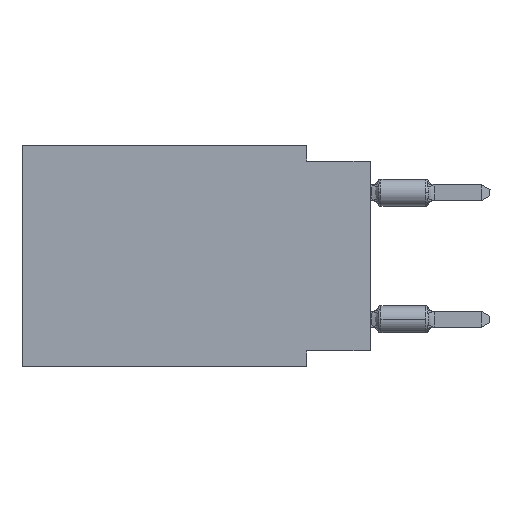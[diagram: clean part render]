
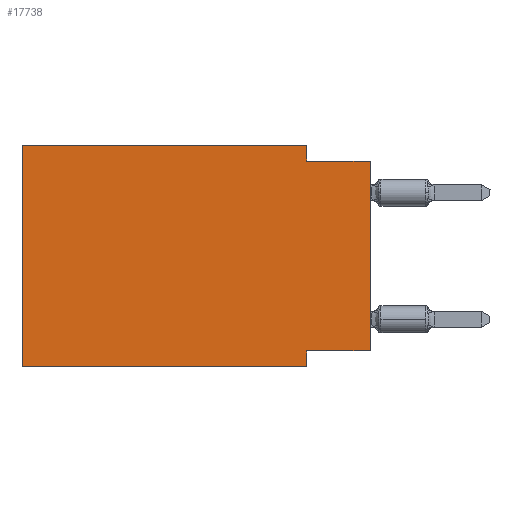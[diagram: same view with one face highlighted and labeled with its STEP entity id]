
A CAD part, left-side view. The second image highlights one B-rep face of the part: STEP entity #17738.
In plain terms, the highlighted planar face has unit normal (-1, 0, 0).
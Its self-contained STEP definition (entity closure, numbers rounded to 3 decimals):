
#125 = CARTESIAN_POINT ( 'NONE',  ( 0., 2.54, -8.89 ) ) ;
#2675 = LINE ( 'NONE', #14570, #33574 ) ;
#3211 = DIRECTION ( 'NONE',  ( 0., -1., 0. ) ) ;
#3425 = EDGE_CURVE ( 'NONE', #47484, #11699, #47341, .T. ) ;
#3649 = EDGE_CURVE ( 'NONE', #46816, #5210, #12224, .T. ) ;
#5210 = VERTEX_POINT ( 'NONE', #11746 ) ;
#6513 = EDGE_CURVE ( 'NONE', #46816, #25596, #2675, .T. ) ;
#7237 = VERTEX_POINT ( 'NONE', #21339 ) ;
#9581 = EDGE_CURVE ( 'NONE', #7237, #25596, #27802, .T. ) ;
#10000 = VECTOR ( 'NONE', #3211, 1000. ) ;
#10481 = CARTESIAN_POINT ( 'NONE',  ( 0., 2.54, 0. ) ) ;
#11631 = CARTESIAN_POINT ( 'NONE',  ( 0., 0., -8.255 ) ) ;
#11699 = VERTEX_POINT ( 'NONE', #10481 ) ;
#11746 = CARTESIAN_POINT ( 'NONE',  ( 0., 2.54, -8.255 ) ) ;
#12224 = LINE ( 'NONE', #53957, #19271 ) ;
#12308 = LINE ( 'NONE', #29142, #48116 ) ;
#14359 = CARTESIAN_POINT ( 'NONE',  ( 0., 2.54, 0. ) ) ;
#14570 = CARTESIAN_POINT ( 'NONE',  ( 0., 0., 0. ) ) ;
#15409 = LINE ( 'NONE', #37204, #41676 ) ;
#16240 = CARTESIAN_POINT ( 'NONE',  ( 0., 13.97, 0. ) ) ;
#17738 = ADVANCED_FACE ( 'NONE', ( #33893 ), #37227, .F. ) ;
#17773 = CARTESIAN_POINT ( 'NONE',  ( 0., 13.97, 0. ) ) ;
#19271 = VECTOR ( 'NONE', #49529, 1000. ) ;
#19993 = ORIENTED_EDGE ( 'NONE', *, *, #3425, .F. ) ;
#21339 = CARTESIAN_POINT ( 'NONE',  ( 0., 2.54, -0.635 ) ) ;
#21587 = VECTOR ( 'NONE', #45179, 1000. ) ;
#21634 = DIRECTION ( 'NONE',  ( 0., -1., 0. ) ) ;
#21737 = CARTESIAN_POINT ( 'NONE',  ( 0., 13.97, 0. ) ) ;
#22059 = ORIENTED_EDGE ( 'NONE', *, *, #54100, .F. ) ;
#23659 = CARTESIAN_POINT ( 'NONE',  ( 0., 0., -0.635 ) ) ;
#23901 = CARTESIAN_POINT ( 'NONE',  ( 0., 13.97, -8.89 ) ) ;
#24892 = VECTOR ( 'NONE', #31481, 1000. ) ;
#25582 = CARTESIAN_POINT ( 'NONE',  ( 0., 0., -0.635 ) ) ;
#25596 = VERTEX_POINT ( 'NONE', #25582 ) ;
#27664 = EDGE_CURVE ( 'NONE', #53916, #47484, #15409, .T. ) ;
#27781 = ORIENTED_EDGE ( 'NONE', *, *, #3649, .F. ) ;
#27802 = LINE ( 'NONE', #23659, #10000 ) ;
#29142 = CARTESIAN_POINT ( 'NONE',  ( 0., 2.54, -8.89 ) ) ;
#29711 = ORIENTED_EDGE ( 'NONE', *, *, #51451, .T. ) ;
#30513 = AXIS2_PLACEMENT_3D ( 'NONE', #16240, #33076, #37775 ) ;
#30667 = LINE ( 'NONE', #14359, #24892 ) ;
#30858 = EDGE_LOOP ( 'NONE', ( #32547, #45887, #48604, #19993, #32117, #29711, #22059, #27781 ) ) ;
#31481 = DIRECTION ( 'NONE',  ( 0., 0., -1. ) ) ;
#32117 = ORIENTED_EDGE ( 'NONE', *, *, #27664, .F. ) ;
#32547 = ORIENTED_EDGE ( 'NONE', *, *, #6513, .T. ) ;
#33076 = DIRECTION ( 'NONE',  ( 1., 0., 0. ) ) ;
#33574 = VECTOR ( 'NONE', #43867, 1000. ) ;
#33893 = FACE_OUTER_BOUND ( 'NONE', #30858, .T. ) ;
#37204 = CARTESIAN_POINT ( 'NONE',  ( 0., 13.97, 0. ) ) ;
#37227 = PLANE ( 'NONE',  #30513 ) ;
#37476 = DIRECTION ( 'NONE',  ( 0., 0., 1. ) ) ;
#37775 = DIRECTION ( 'NONE',  ( 0., 0., -1. ) ) ;
#40202 = EDGE_CURVE ( 'NONE', #11699, #7237, #30667, .T. ) ;
#41303 = CARTESIAN_POINT ( 'NONE',  ( 0., 13.97, -8.89 ) ) ;
#41676 = VECTOR ( 'NONE', #37476, 1000. ) ;
#43867 = DIRECTION ( 'NONE',  ( 0., 0., 1. ) ) ;
#45179 = DIRECTION ( 'NONE',  ( 0., -1., 0. ) ) ;
#45887 = ORIENTED_EDGE ( 'NONE', *, *, #9581, .F. ) ;
#46816 = VERTEX_POINT ( 'NONE', #11631 ) ;
#47341 = LINE ( 'NONE', #17773, #50029 ) ;
#47484 = VERTEX_POINT ( 'NONE', #21737 ) ;
#47767 = VERTEX_POINT ( 'NONE', #125 ) ;
#48116 = VECTOR ( 'NONE', #51242, 1000. ) ;
#48604 = ORIENTED_EDGE ( 'NONE', *, *, #40202, .F. ) ;
#49529 = DIRECTION ( 'NONE',  ( 0., 1., 0. ) ) ;
#50029 = VECTOR ( 'NONE', #21634, 1000. ) ;
#51242 = DIRECTION ( 'NONE',  ( 0., 0., -1. ) ) ;
#51451 = EDGE_CURVE ( 'NONE', #53916, #47767, #53763, .T. ) ;
#53763 = LINE ( 'NONE', #41303, #21587 ) ;
#53916 = VERTEX_POINT ( 'NONE', #23901 ) ;
#53957 = CARTESIAN_POINT ( 'NONE',  ( 0., 0., -8.255 ) ) ;
#54100 = EDGE_CURVE ( 'NONE', #5210, #47767, #12308, .T. ) ;
